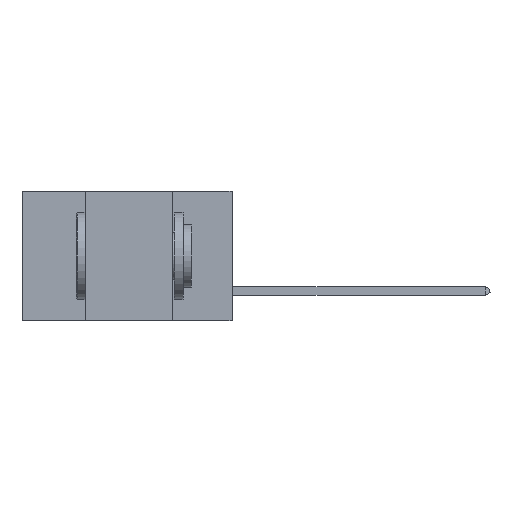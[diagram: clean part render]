
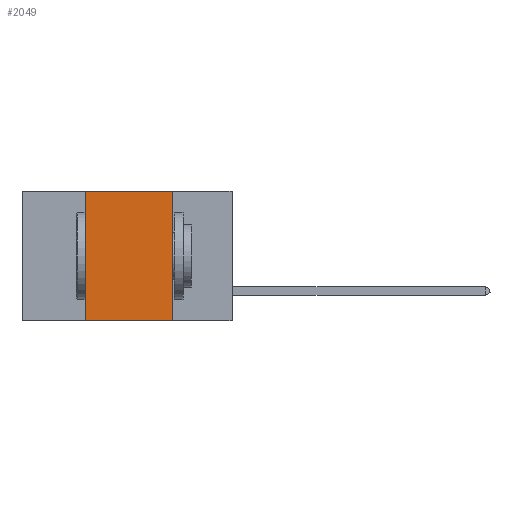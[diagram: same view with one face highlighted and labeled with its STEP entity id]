
A CAD part, left-side view. The second image highlights one B-rep face of the part: STEP entity #2049.
In plain terms, the highlighted planar face has unit normal (-1, 0, 0).
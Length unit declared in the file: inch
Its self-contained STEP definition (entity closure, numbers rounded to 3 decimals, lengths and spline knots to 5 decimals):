
#140 = VECTOR ( 'NONE', #38164, 39.37008 ) ;
#851 = VECTOR ( 'NONE', #22333, 39.37008 ) ;
#1009 = VERTEX_POINT ( 'NONE', #14316 ) ;
#2049 = ADVANCED_FACE ( 'NONE', ( #24161 ), #15568, .F. ) ;
#2841 = AXIS2_PLACEMENT_3D ( 'NONE', #19511, #11758, #47039 ) ;
#3796 = DIRECTION ( 'NONE',  ( 0., 0., 1. ) ) ;
#4329 = LINE ( 'NONE', #15764, #13512 ) ;
#4726 = EDGE_LOOP ( 'NONE', ( #10650, #25310, #26268, #36434 ) ) ;
#7324 = VERTEX_POINT ( 'NONE', #7749 ) ;
#7749 = CARTESIAN_POINT ( 'NONE',  ( 0., 0.42, -0.37 ) ) ;
#10650 = ORIENTED_EDGE ( 'NONE', *, *, #13275, .F. ) ;
#11758 = DIRECTION ( 'NONE',  ( 1., 0., 0. ) ) ;
#11783 = LINE ( 'NONE', #49707, #140 ) ;
#11961 = DIRECTION ( 'NONE',  ( 0., -1., 0. ) ) ;
#13275 = EDGE_CURVE ( 'NONE', #30500, #43277, #11783, .T. ) ;
#13512 = VECTOR ( 'NONE', #11961, 39.37008 ) ;
#14316 = CARTESIAN_POINT ( 'NONE',  ( 0., 0.42, 0. ) ) ;
#14422 = LINE ( 'NONE', #50559, #28583 ) ;
#15568 = PLANE ( 'NONE',  #2841 ) ;
#15764 = CARTESIAN_POINT ( 'NONE',  ( 0., 0.6, -0.37 ) ) ;
#19511 = CARTESIAN_POINT ( 'NONE',  ( 0., 0.6, 0. ) ) ;
#22333 = DIRECTION ( 'NONE',  ( 0., -1., 0. ) ) ;
#24161 = FACE_OUTER_BOUND ( 'NONE', #4726, .T. ) ;
#25310 = ORIENTED_EDGE ( 'NONE', *, *, #32330, .F. ) ;
#26268 = ORIENTED_EDGE ( 'NONE', *, *, #28045, .F. ) ;
#26289 = CARTESIAN_POINT ( 'NONE',  ( 0., 0.17, 0. ) ) ;
#28045 = EDGE_CURVE ( 'NONE', #7324, #1009, #14422, .T. ) ;
#28583 = VECTOR ( 'NONE', #3796, 39.37008 ) ;
#30500 = VERTEX_POINT ( 'NONE', #26289 ) ;
#30779 = EDGE_CURVE ( 'NONE', #7324, #43277, #4329, .T. ) ;
#32330 = EDGE_CURVE ( 'NONE', #1009, #30500, #32781, .T. ) ;
#32781 = LINE ( 'NONE', #34698, #851 ) ;
#34698 = CARTESIAN_POINT ( 'NONE',  ( 0., 0.6, 0. ) ) ;
#36434 = ORIENTED_EDGE ( 'NONE', *, *, #30779, .T. ) ;
#38164 = DIRECTION ( 'NONE',  ( 0., 0., -1. ) ) ;
#43277 = VERTEX_POINT ( 'NONE', #47207 ) ;
#47039 = DIRECTION ( 'NONE',  ( 0., 0., -1. ) ) ;
#47207 = CARTESIAN_POINT ( 'NONE',  ( 0., 0.17, -0.37 ) ) ;
#49707 = CARTESIAN_POINT ( 'NONE',  ( 0., 0.17, 0. ) ) ;
#50559 = CARTESIAN_POINT ( 'NONE',  ( 0., 0.42, 0. ) ) ;
